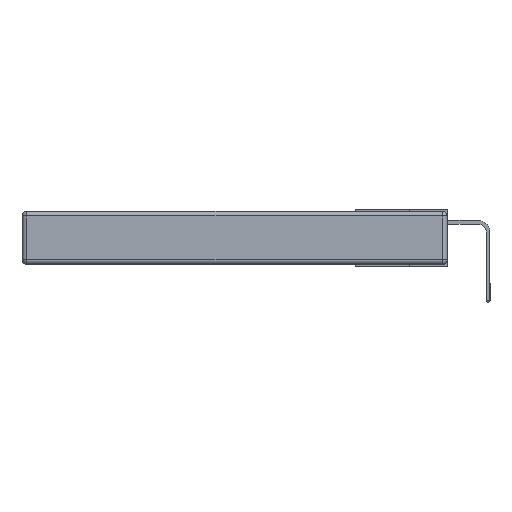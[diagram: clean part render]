
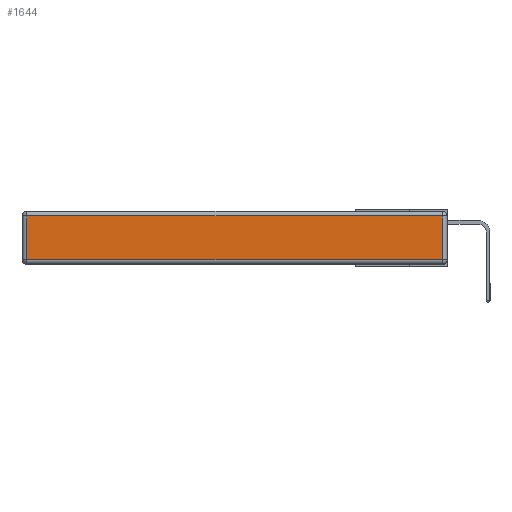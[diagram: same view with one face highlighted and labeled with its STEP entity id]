
A CAD part, left-side view. The second image highlights one B-rep face of the part: STEP entity #1644.
In plain terms, the highlighted planar face has unit normal (-1, 0, 0).
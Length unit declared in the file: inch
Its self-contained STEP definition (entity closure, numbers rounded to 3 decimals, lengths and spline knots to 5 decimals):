
#211 = ORIENTED_EDGE ( 'NONE', *, *, #542, .T. ) ;
#542 = EDGE_CURVE ( 'NONE', #10769, #6691, #7600, .T. ) ;
#869 = CARTESIAN_POINT ( 'NONE',  ( 0., 0.03, -0.03 ) ) ;
#1159 = CARTESIAN_POINT ( 'NONE',  ( 0., 2.72, -0.03 ) ) ;
#1463 = PLANE ( 'NONE',  #2543 ) ;
#1644 = ADVANCED_FACE ( 'NONE', ( #10787 ), #1463, .T. ) ;
#2008 = DIRECTION ( 'NONE',  ( 0., 0., 1. ) ) ;
#2022 = VERTEX_POINT ( 'NONE', #869 ) ;
#2446 = EDGE_CURVE ( 'NONE', #2022, #4081, #9759, .T. ) ;
#2543 = AXIS2_PLACEMENT_3D ( 'NONE', #12661, #6376, #7440 ) ;
#2778 = CARTESIAN_POINT ( 'NONE',  ( 0., 2.75, -0.03 ) ) ;
#3243 = VECTOR ( 'NONE', #7166, 39.37008 ) ;
#4081 = VERTEX_POINT ( 'NONE', #1159 ) ;
#5884 = DIRECTION ( 'NONE',  ( 0., 1., 0. ) ) ;
#6376 = DIRECTION ( 'NONE',  ( -1., 0., 0. ) ) ;
#6691 = VERTEX_POINT ( 'NONE', #12737 ) ;
#7088 = LINE ( 'NONE', #12444, #3243 ) ;
#7166 = DIRECTION ( 'NONE',  ( 0., 0., -1. ) ) ;
#7440 = DIRECTION ( 'NONE',  ( 0., 0., 1. ) ) ;
#7600 = LINE ( 'NONE', #10973, #11943 ) ;
#7978 = ORIENTED_EDGE ( 'NONE', *, *, #2446, .T. ) ;
#8495 = LINE ( 'NONE', #13611, #10846 ) ;
#8550 = ORIENTED_EDGE ( 'NONE', *, *, #12696, .T. ) ;
#9759 = LINE ( 'NONE', #2778, #12262 ) ;
#9886 = CARTESIAN_POINT ( 'NONE',  ( 0., 2.72, -0.313 ) ) ;
#10319 = ORIENTED_EDGE ( 'NONE', *, *, #13493, .T. ) ;
#10514 = EDGE_LOOP ( 'NONE', ( #211, #10319, #7978, #8550 ) ) ;
#10769 = VERTEX_POINT ( 'NONE', #9886 ) ;
#10787 = FACE_OUTER_BOUND ( 'NONE', #10514, .T. ) ;
#10846 = VECTOR ( 'NONE', #2008, 39.37008 ) ;
#10973 = CARTESIAN_POINT ( 'NONE',  ( 0., 0., -0.313 ) ) ;
#11943 = VECTOR ( 'NONE', #12030, 39.37008 ) ;
#12030 = DIRECTION ( 'NONE',  ( 0., -1., 0. ) ) ;
#12262 = VECTOR ( 'NONE', #5884, 39.37008 ) ;
#12444 = CARTESIAN_POINT ( 'NONE',  ( 0., 2.72, -0.343 ) ) ;
#12661 = CARTESIAN_POINT ( 'NONE',  ( 0., 0., -0.343 ) ) ;
#12696 = EDGE_CURVE ( 'NONE', #4081, #10769, #7088, .T. ) ;
#12737 = CARTESIAN_POINT ( 'NONE',  ( 0., 0.03, -0.313 ) ) ;
#13493 = EDGE_CURVE ( 'NONE', #6691, #2022, #8495, .T. ) ;
#13611 = CARTESIAN_POINT ( 'NONE',  ( 0., 0.03, -0.343 ) ) ;
